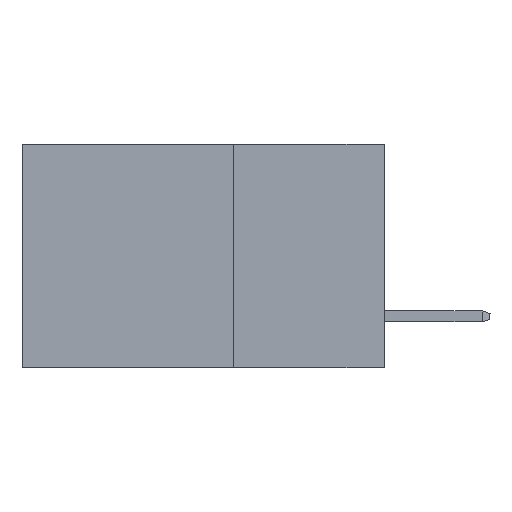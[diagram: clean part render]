
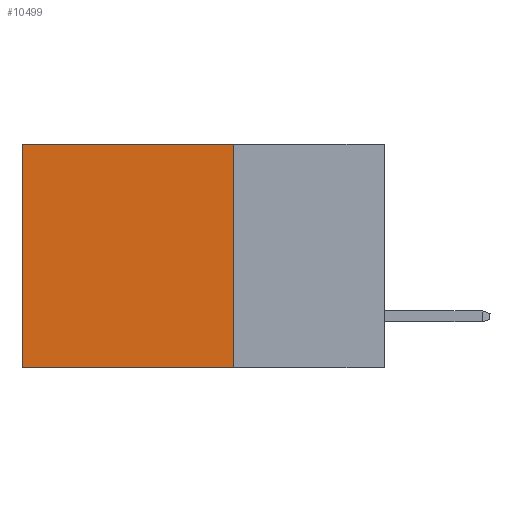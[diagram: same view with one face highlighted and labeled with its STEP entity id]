
A CAD part, left-side view. The second image highlights one B-rep face of the part: STEP entity #10499.
In plain terms, the highlighted planar face has unit normal (-1, 0, 0).
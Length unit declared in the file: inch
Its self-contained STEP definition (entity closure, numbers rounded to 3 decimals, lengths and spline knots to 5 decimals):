
#59 = ORIENTED_EDGE ( 'NONE', *, *, #1257, .F. ) ;
#196 = CARTESIAN_POINT ( 'NONE',  ( 0.2615, 0.25, -0.37 ) ) ;
#238 = CARTESIAN_POINT ( 'NONE',  ( 0.2615, 0.6, -0.37 ) ) ;
#485 = VECTOR ( 'NONE', #2415, 39.37008 ) ;
#643 = VERTEX_POINT ( 'NONE', #7286 ) ;
#1119 = VECTOR ( 'NONE', #2054, 39.37008 ) ;
#1257 = EDGE_CURVE ( 'NONE', #6868, #1786, #1954, .T. ) ;
#1259 = ORIENTED_EDGE ( 'NONE', *, *, #2090, .T. ) ;
#1483 = VECTOR ( 'NONE', #1878, 39.37008 ) ;
#1589 = LINE ( 'NONE', #10012, #485 ) ;
#1786 = VERTEX_POINT ( 'NONE', #10511 ) ;
#1878 = DIRECTION ( 'NONE',  ( 0., 1., 0. ) ) ;
#1954 = LINE ( 'NONE', #196, #1119 ) ;
#2054 = DIRECTION ( 'NONE',  ( 0., 0., -1. ) ) ;
#2090 = EDGE_CURVE ( 'NONE', #6868, #2748, #7789, .T. ) ;
#2134 = AXIS2_PLACEMENT_3D ( 'NONE', #7448, #3222, #10773 ) ;
#2415 = DIRECTION ( 'NONE',  ( 0., 1., 0. ) ) ;
#2748 = VERTEX_POINT ( 'NONE', #8842 ) ;
#2833 = CARTESIAN_POINT ( 'NONE',  ( 0.2615, 0.25, 0. ) ) ;
#3040 = EDGE_CURVE ( 'NONE', #2748, #643, #4518, .T. ) ;
#3222 = DIRECTION ( 'NONE',  ( 1., 0., 0. ) ) ;
#3997 = FACE_OUTER_BOUND ( 'NONE', #5858, .T. ) ;
#4518 = LINE ( 'NONE', #238, #6773 ) ;
#5383 = CARTESIAN_POINT ( 'NONE',  ( 0.2615, 0.25, 0. ) ) ;
#5481 = EDGE_CURVE ( 'NONE', #1786, #643, #1589, .T. ) ;
#5634 = PLANE ( 'NONE',  #2134 ) ;
#5858 = EDGE_LOOP ( 'NONE', ( #9770, #7113, #59, #1259 ) ) ;
#6773 = VECTOR ( 'NONE', #8729, 39.37008 ) ;
#6868 = VERTEX_POINT ( 'NONE', #2833 ) ;
#7113 = ORIENTED_EDGE ( 'NONE', *, *, #5481, .F. ) ;
#7286 = CARTESIAN_POINT ( 'NONE',  ( 0.2615, 0.6, -0.37 ) ) ;
#7448 = CARTESIAN_POINT ( 'NONE',  ( 0.2615, 0.25, -0.37 ) ) ;
#7789 = LINE ( 'NONE', #5383, #1483 ) ;
#8729 = DIRECTION ( 'NONE',  ( 0., 0., -1. ) ) ;
#8842 = CARTESIAN_POINT ( 'NONE',  ( 0.2615, 0.6, 0. ) ) ;
#9770 = ORIENTED_EDGE ( 'NONE', *, *, #3040, .T. ) ;
#10012 = CARTESIAN_POINT ( 'NONE',  ( 0.2615, 0.25, -0.37 ) ) ;
#10499 = ADVANCED_FACE ( 'NONE', ( #3997 ), #5634, .F. ) ;
#10511 = CARTESIAN_POINT ( 'NONE',  ( 0.2615, 0.25, -0.37 ) ) ;
#10773 = DIRECTION ( 'NONE',  ( 0., 0., -1. ) ) ;
